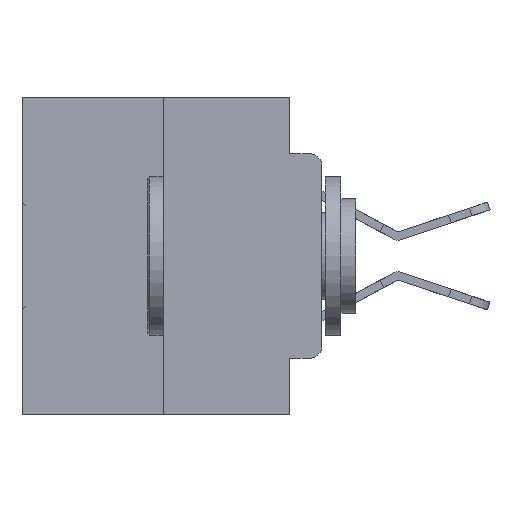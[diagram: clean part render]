
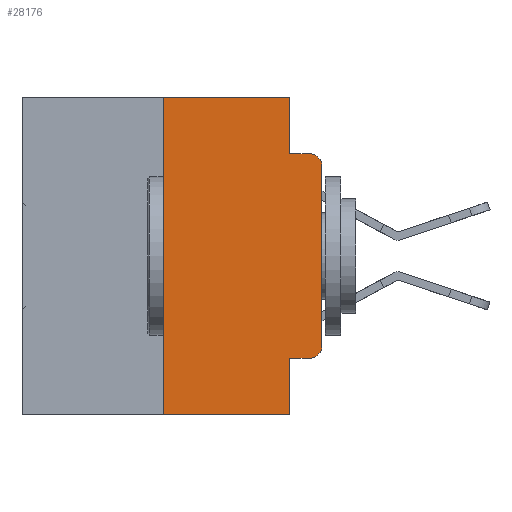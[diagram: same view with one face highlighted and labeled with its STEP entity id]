
A CAD part, left-side view. The second image highlights one B-rep face of the part: STEP entity #28176.
In plain terms, the highlighted planar face has unit normal (-1, 0, 0).
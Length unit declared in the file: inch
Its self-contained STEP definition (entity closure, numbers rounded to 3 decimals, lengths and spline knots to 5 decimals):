
#597 = ORIENTED_EDGE ( 'NONE', *, *, #12457, .F. ) ;
#1191 = VERTEX_POINT ( 'NONE', #28863 ) ;
#1459 = CARTESIAN_POINT ( 'NONE',  ( 0., 0.051, 0. ) ) ;
#1468 = CARTESIAN_POINT ( 'NONE',  ( 0., 0.051, -0.4115 ) ) ;
#1482 = DIRECTION ( 'NONE',  ( 0., 0., 1. ) ) ;
#1810 = DIRECTION ( 'NONE',  ( 0., 0., 1. ) ) ;
#2257 = DIRECTION ( 'NONE',  ( 0., -1., 0. ) ) ;
#2274 = CARTESIAN_POINT ( 'NONE',  ( 0., 0.25, -0.5 ) ) ;
#2336 = VERTEX_POINT ( 'NONE', #29711 ) ;
#2434 = VECTOR ( 'NONE', #8460, 39.37008 ) ;
#2700 = LINE ( 'NONE', #23787, #2434 ) ;
#3479 = EDGE_CURVE ( 'NONE', #1191, #16410, #2700, .T. ) ;
#3630 = EDGE_CURVE ( 'NONE', #19609, #1191, #6399, .T. ) ;
#4279 = LINE ( 'NONE', #6319, #9050 ) ;
#4671 = DIRECTION ( 'NONE',  ( 0., 0., -1. ) ) ;
#5412 = VERTEX_POINT ( 'NONE', #8444 ) ;
#5769 = VECTOR ( 'NONE', #1810, 39.37008 ) ;
#6319 = CARTESIAN_POINT ( 'NONE',  ( 0., 0.473, -0.5 ) ) ;
#6399 = LINE ( 'NONE', #1459, #23762 ) ;
#6410 = LINE ( 'NONE', #9646, #5769 ) ;
#6505 = LINE ( 'NONE', #19274, #27705 ) ;
#7565 = DIRECTION ( 'NONE',  ( 0., 0., -1. ) ) ;
#8444 = CARTESIAN_POINT ( 'NONE',  ( 0., 0.051, -0.5 ) ) ;
#8460 = DIRECTION ( 'NONE',  ( 0., -1., 0. ) ) ;
#8633 = VECTOR ( 'NONE', #2257, 39.37008 ) ;
#9050 = VECTOR ( 'NONE', #14650, 39.37008 ) ;
#9321 = CARTESIAN_POINT ( 'NONE',  ( 0., 0., -0.1085 ) ) ;
#9646 = CARTESIAN_POINT ( 'NONE',  ( 0., 0.25, 0. ) ) ;
#10057 = DIRECTION ( 'NONE',  ( -1., 0., 0. ) ) ;
#10116 = FACE_OUTER_BOUND ( 'NONE', #21741, .T. ) ;
#10471 = CARTESIAN_POINT ( 'NONE',  ( 0., 0.02, -0.0885 ) ) ;
#10638 = VECTOR ( 'NONE', #19691, 39.37008 ) ;
#12157 = VERTEX_POINT ( 'NONE', #27749 ) ;
#12457 = EDGE_CURVE ( 'NONE', #12157, #5412, #6505, .T. ) ;
#13830 = DIRECTION ( 'NONE',  ( 0., 0., -1. ) ) ;
#14230 = ORIENTED_EDGE ( 'NONE', *, *, #16255, .T. ) ;
#14237 = CARTESIAN_POINT ( 'NONE',  ( 0., 0., 0. ) ) ;
#14650 = DIRECTION ( 'NONE',  ( 0., -1., 0. ) ) ;
#15526 = EDGE_CURVE ( 'NONE', #20390, #16360, #18200, .T. ) ;
#16255 = EDGE_CURVE ( 'NONE', #12157, #20390, #29731, .T. ) ;
#16292 = EDGE_CURVE ( 'NONE', #25384, #2336, #6410, .T. ) ;
#16360 = VERTEX_POINT ( 'NONE', #28360 ) ;
#16410 = VERTEX_POINT ( 'NONE', #10471 ) ;
#18200 = CIRCLE ( 'NONE', #29604, 0.02 ) ;
#19191 = LINE ( 'NONE', #14237, #31275 ) ;
#19274 = CARTESIAN_POINT ( 'NONE',  ( 0., 0.051, 0. ) ) ;
#19609 = VERTEX_POINT ( 'NONE', #28999 ) ;
#19656 = EDGE_CURVE ( 'NONE', #25384, #5412, #4279, .T. ) ;
#19691 = DIRECTION ( 'NONE',  ( 0., -1., 0. ) ) ;
#20004 = CARTESIAN_POINT ( 'NONE',  ( 0., 0.02, -0.1085 ) ) ;
#20146 = LINE ( 'NONE', #33215, #8633 ) ;
#20390 = VERTEX_POINT ( 'NONE', #23956 ) ;
#20503 = PLANE ( 'NONE',  #24282 ) ;
#21741 = EDGE_LOOP ( 'NONE', ( #26101, #23093, #31897, #24089, #30103, #26385, #28938, #597, #14230, #33252 ) ) ;
#23093 = ORIENTED_EDGE ( 'NONE', *, *, #25142, .T. ) ;
#23762 = VECTOR ( 'NONE', #27509, 39.37008 ) ;
#23787 = CARTESIAN_POINT ( 'NONE',  ( 0., 0.051, -0.0885 ) ) ;
#23956 = CARTESIAN_POINT ( 'NONE',  ( 0., 0.02, -0.4115 ) ) ;
#24089 = ORIENTED_EDGE ( 'NONE', *, *, #3630, .F. ) ;
#24282 = AXIS2_PLACEMENT_3D ( 'NONE', #25092, #30877, #7565 ) ;
#24734 = DIRECTION ( 'NONE',  ( -1., 0., 0. ) ) ;
#25092 = CARTESIAN_POINT ( 'NONE',  ( 0., 0.473, 0. ) ) ;
#25142 = EDGE_CURVE ( 'NONE', #29380, #16410, #27763, .T. ) ;
#25384 = VERTEX_POINT ( 'NONE', #2274 ) ;
#26101 = ORIENTED_EDGE ( 'NONE', *, *, #31332, .T. ) ;
#26385 = ORIENTED_EDGE ( 'NONE', *, *, #16292, .F. ) ;
#26698 = AXIS2_PLACEMENT_3D ( 'NONE', #20004, #24734, #4671 ) ;
#27509 = DIRECTION ( 'NONE',  ( 0., 0., -1. ) ) ;
#27705 = VECTOR ( 'NONE', #13830, 39.37008 ) ;
#27749 = CARTESIAN_POINT ( 'NONE',  ( 0., 0.051, -0.4115 ) ) ;
#27763 = CIRCLE ( 'NONE', #26698, 0.02 ) ;
#28176 = ADVANCED_FACE ( 'NONE', ( #10116 ), #20503, .F. ) ;
#28360 = CARTESIAN_POINT ( 'NONE',  ( 0., 0., -0.3915 ) ) ;
#28863 = CARTESIAN_POINT ( 'NONE',  ( 0., 0.051, -0.0885 ) ) ;
#28938 = ORIENTED_EDGE ( 'NONE', *, *, #19656, .T. ) ;
#28999 = CARTESIAN_POINT ( 'NONE',  ( 0., 0.051, 0. ) ) ;
#29380 = VERTEX_POINT ( 'NONE', #9321 ) ;
#29604 = AXIS2_PLACEMENT_3D ( 'NONE', #33348, #10057, #33529 ) ;
#29711 = CARTESIAN_POINT ( 'NONE',  ( 0., 0.25, 0. ) ) ;
#29731 = LINE ( 'NONE', #1468, #10638 ) ;
#29844 = EDGE_CURVE ( 'NONE', #2336, #19609, #20146, .T. ) ;
#30103 = ORIENTED_EDGE ( 'NONE', *, *, #29844, .F. ) ;
#30877 = DIRECTION ( 'NONE',  ( 1., 0., 0. ) ) ;
#31275 = VECTOR ( 'NONE', #1482, 39.37008 ) ;
#31332 = EDGE_CURVE ( 'NONE', #16360, #29380, #19191, .T. ) ;
#31897 = ORIENTED_EDGE ( 'NONE', *, *, #3479, .F. ) ;
#33215 = CARTESIAN_POINT ( 'NONE',  ( 0., 0.473, 0. ) ) ;
#33252 = ORIENTED_EDGE ( 'NONE', *, *, #15526, .T. ) ;
#33348 = CARTESIAN_POINT ( 'NONE',  ( 0., 0.02, -0.3915 ) ) ;
#33529 = DIRECTION ( 'NONE',  ( 0., 0., -1. ) ) ;
